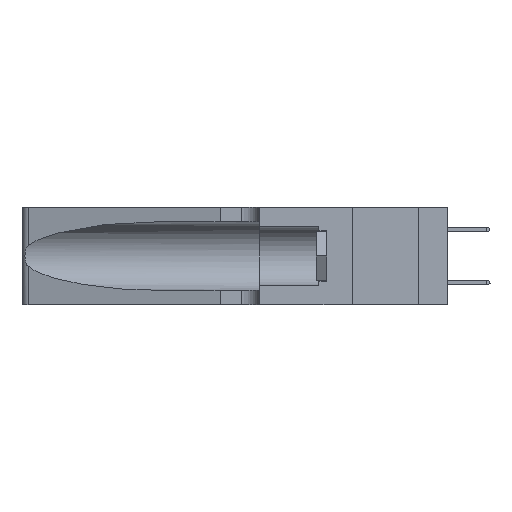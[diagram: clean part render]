
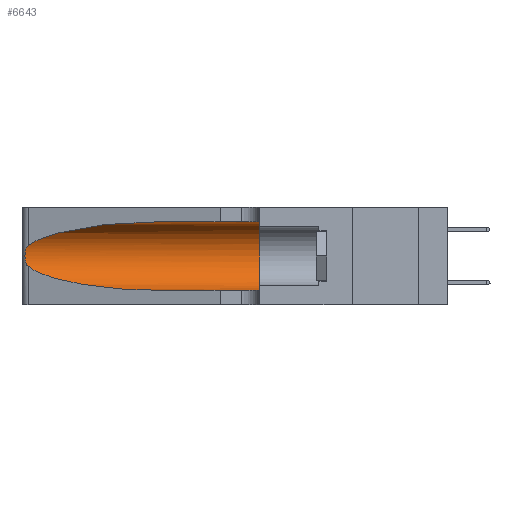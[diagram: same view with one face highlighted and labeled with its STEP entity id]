
A CAD part, left-side view. The second image highlights one B-rep face of the part: STEP entity #6643.
In plain terms, the highlighted cylindrical face has radius 3.308 mm (diameter 6.617 mm), a partial arc.
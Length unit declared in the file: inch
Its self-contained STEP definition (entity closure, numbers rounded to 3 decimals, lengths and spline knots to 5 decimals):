
#357 = VERTEX_POINT ( 'NONE', #20261 ) ;
#2229 = CARTESIAN_POINT ( 'NONE',  ( 0.25555, 1.22994, 0.2215 ) ) ;
#2638 = CARTESIAN_POINT ( 'NONE',  ( 0.26075, 1.23896, 0.178 ) ) ;
#2720 = VECTOR ( 'NONE', #4880, 39.37008 ) ;
#3697 = B_SPLINE_CURVE_WITH_KNOTS ( 'NONE', 3,
 ( #7804, #2229, #5358, #15219, #37005, #9172, #18202, #2638, #18740, #21612, #31118, #37272, #12311, #18343 ),
 .UNSPECIFIED., .F., .F.,
 ( 4, 2, 2, 2, 2, 2, 4 ),
 ( 0., 0.00027, 0.00053, 0.00107, 0.0016, 0.00187, 0.00214 ),
 .UNSPECIFIED. ) ;
#4880 = DIRECTION ( 'NONE',  ( 0., -1., 0. ) ) ;
#5126 = CARTESIAN_POINT ( 'NONE',  ( 0.1305, 1.61858, 0.185 ) ) ;
#5358 = CARTESIAN_POINT ( 'NONE',  ( 0.25639, 1.23184, 0.21858 ) ) ;
#6643 = ADVANCED_FACE ( 'NONE', ( #13490 ), #24315, .F. ) ;
#6958 = VECTOR ( 'NONE', #34188, 39.37008 ) ;
#7254 = DIRECTION ( 'NONE',  ( 0., 1., 0. ) ) ;
#7804 = CARTESIAN_POINT ( 'NONE',  ( 0.25487, 1.22718, 0.22369 ) ) ;
#8922 = EDGE_CURVE ( 'NONE', #10738, #357, #22011, .T. ) ;
#9172 = CARTESIAN_POINT ( 'NONE',  ( 0.26018, 1.23835, 0.19895 ) ) ;
#9239 =( BOUNDED_CURVE ( )  B_SPLINE_CURVE ( 3, ( #13100, #37807, #35047, #19011 ),
 .UNSPECIFIED., .F., .F. ) 
 B_SPLINE_CURVE_WITH_KNOTS ( ( 4, 4 ),
 ( 3.44316, 4.71239 ),
 .UNSPECIFIED. ) 
 CURVE ( )  GEOMETRIC_REPRESENTATION_ITEM ( )  RATIONAL_B_SPLINE_CURVE ( ( 1., 0.87, 0.87, 1. ) ) 
 REPRESENTATION_ITEM ( '' )  );
#10738 = VERTEX_POINT ( 'NONE', #30703 ) ;
#12311 = CARTESIAN_POINT ( 'NONE',  ( 0.25555, 1.22993, 0.14849 ) ) ;
#13100 = CARTESIAN_POINT ( 'NONE',  ( 0.25487, 1.22718, 0.14631 ) ) ;
#13375 = LINE ( 'NONE', #24584, #6958 ) ;
#13490 = FACE_OUTER_BOUND ( 'NONE', #28026, .T. ) ;
#13701 = EDGE_CURVE ( 'NONE', #357, #35460, #3697, .T. ) ;
#15219 = CARTESIAN_POINT ( 'NONE',  ( 0.25787, 1.23484, 0.2124 ) ) ;
#16127 = VERTEX_POINT ( 'NONE', #25184 ) ;
#18085 = VERTEX_POINT ( 'NONE', #38576 ) ;
#18202 = CARTESIAN_POINT ( 'NONE',  ( 0.26075, 1.23896, 0.19203 ) ) ;
#18343 = CARTESIAN_POINT ( 'NONE',  ( 0.25487, 1.22718, 0.14631 ) ) ;
#18347 = ORIENTED_EDGE ( 'NONE', *, *, #29359, .F. ) ;
#18740 = CARTESIAN_POINT ( 'NONE',  ( 0.26017, 1.23833, 0.17102 ) ) ;
#19011 = CARTESIAN_POINT ( 'NONE',  ( 0.1305, 0.72297, 0.05475 ) ) ;
#20261 = CARTESIAN_POINT ( 'NONE',  ( 0.25487, 1.22718, 0.22369 ) ) ;
#20572 = DIRECTION ( 'NONE',  ( 0., 0., -1. ) ) ;
#20632 = CARTESIAN_POINT ( 'NONE',  ( 0.1305, 0.72297, 0.05475 ) ) ;
#21194 = VERTEX_POINT ( 'NONE', #20632 ) ;
#21424 = EDGE_CURVE ( 'NONE', #16127, #18085, #22316, .T. ) ;
#21612 = CARTESIAN_POINT ( 'NONE',  ( 0.25856, 1.23593, 0.16098 ) ) ;
#22011 =( BOUNDED_CURVE ( )  B_SPLINE_CURVE ( 3, ( #32941, #27324, #24174, #31300 ),
 .UNSPECIFIED., .F., .T. ) 
 B_SPLINE_CURVE_WITH_KNOTS ( ( 4, 4 ),
 ( 1.5708, 2.84003 ),
 .UNSPECIFIED. ) 
 CURVE ( )  GEOMETRIC_REPRESENTATION_ITEM ( )  RATIONAL_B_SPLINE_CURVE ( ( 1., 0.87, 0.87, 1. ) ) 
 REPRESENTATION_ITEM ( '' )  );
#22316 = CIRCLE ( 'NONE', #29489, 0.13025 ) ;
#22730 = CARTESIAN_POINT ( 'NONE',  ( 0.1305, 0.35, 0.185 ) ) ;
#24174 = CARTESIAN_POINT ( 'NONE',  ( 0.2373, 1.15595, 0.28018 ) ) ;
#24315 = CYLINDRICAL_SURFACE ( 'NONE', #34656, 0.13025 ) ;
#24584 = CARTESIAN_POINT ( 'NONE',  ( 0.1305, 1.61858, 0.31525 ) ) ;
#25184 = CARTESIAN_POINT ( 'NONE',  ( 0.1305, 0.35, 0.31525 ) ) ;
#26072 = DIRECTION ( 'NONE',  ( 0., 0., 1. ) ) ;
#26685 = DIRECTION ( 'NONE',  ( 0., -1., 0. ) ) ;
#27324 = CARTESIAN_POINT ( 'NONE',  ( 0.18966, 0.96281, 0.31525 ) ) ;
#28026 = EDGE_LOOP ( 'NONE', ( #40452, #33016, #31065, #39941, #29144, #18347 ) ) ;
#28298 = EDGE_CURVE ( 'NONE', #35460, #21194, #9239, .T. ) ;
#29144 = ORIENTED_EDGE ( 'NONE', *, *, #21424, .F. ) ;
#29265 = EDGE_CURVE ( 'NONE', #21194, #18085, #35488, .T. ) ;
#29359 = EDGE_CURVE ( 'NONE', #10738, #16127, #13375, .T. ) ;
#29489 = AXIS2_PLACEMENT_3D ( 'NONE', #22730, #7254, #26072 ) ;
#29727 = CARTESIAN_POINT ( 'NONE',  ( 0.25487, 1.22718, 0.14631 ) ) ;
#30127 = CARTESIAN_POINT ( 'NONE',  ( 0.1305, 1.61858, 0.05475 ) ) ;
#30703 = CARTESIAN_POINT ( 'NONE',  ( 0.1305, 0.72297, 0.31525 ) ) ;
#31065 = ORIENTED_EDGE ( 'NONE', *, *, #28298, .T. ) ;
#31118 = CARTESIAN_POINT ( 'NONE',  ( 0.25789, 1.23486, 0.15765 ) ) ;
#31300 = CARTESIAN_POINT ( 'NONE',  ( 0.25487, 1.22718, 0.22369 ) ) ;
#32941 = CARTESIAN_POINT ( 'NONE',  ( 0.1305, 0.72297, 0.31525 ) ) ;
#33016 = ORIENTED_EDGE ( 'NONE', *, *, #13701, .T. ) ;
#34188 = DIRECTION ( 'NONE',  ( 0., -1., 0. ) ) ;
#34656 = AXIS2_PLACEMENT_3D ( 'NONE', #5126, #26685, #20572 ) ;
#35047 = CARTESIAN_POINT ( 'NONE',  ( 0.18966, 0.96281, 0.05475 ) ) ;
#35460 = VERTEX_POINT ( 'NONE', #29727 ) ;
#35488 = LINE ( 'NONE', #30127, #2720 ) ;
#37005 = CARTESIAN_POINT ( 'NONE',  ( 0.25854, 1.2359, 0.20912 ) ) ;
#37272 = CARTESIAN_POINT ( 'NONE',  ( 0.25639, 1.23186, 0.15144 ) ) ;
#37807 = CARTESIAN_POINT ( 'NONE',  ( 0.2373, 1.15595, 0.08982 ) ) ;
#38576 = CARTESIAN_POINT ( 'NONE',  ( 0.1305, 0.35, 0.05475 ) ) ;
#39941 = ORIENTED_EDGE ( 'NONE', *, *, #29265, .T. ) ;
#40452 = ORIENTED_EDGE ( 'NONE', *, *, #8922, .T. ) ;
